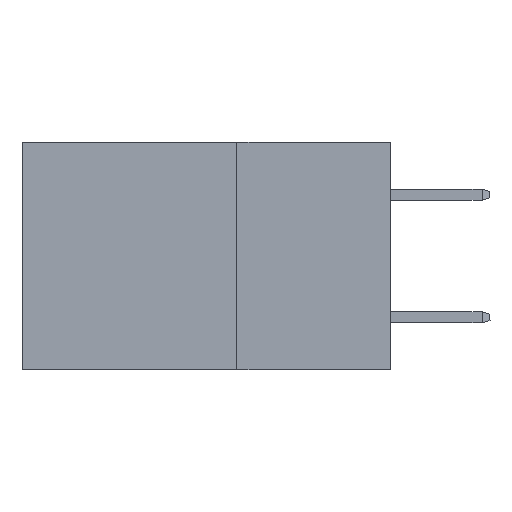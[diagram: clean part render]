
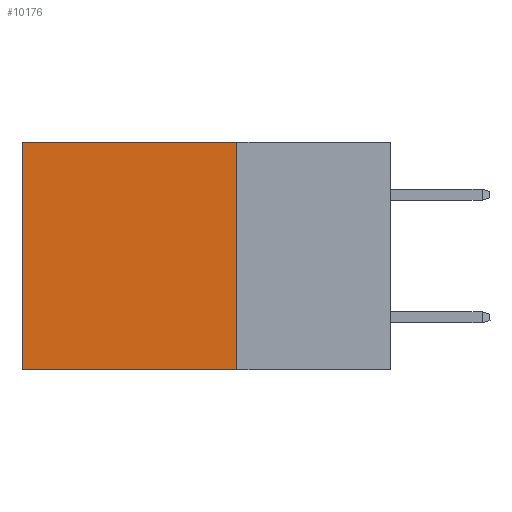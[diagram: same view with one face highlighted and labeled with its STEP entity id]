
A CAD part, left-side view. The second image highlights one B-rep face of the part: STEP entity #10176.
In plain terms, the highlighted planar face has unit normal (-1, 0, 0).
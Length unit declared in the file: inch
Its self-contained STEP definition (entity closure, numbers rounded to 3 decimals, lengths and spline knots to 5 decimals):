
#93 = VERTEX_POINT ( 'NONE', #11390 ) ;
#306 = VECTOR ( 'NONE', #2499, 39.37008 ) ;
#409 = EDGE_LOOP ( 'NONE', ( #2734, #11224, #6545, #11373 ) ) ;
#805 = LINE ( 'NONE', #5306, #1109 ) ;
#1109 = VECTOR ( 'NONE', #12263, 39.37008 ) ;
#1294 = VERTEX_POINT ( 'NONE', #9379 ) ;
#1542 = CARTESIAN_POINT ( 'NONE',  ( 0.2875, 0.6, 0. ) ) ;
#1719 = VECTOR ( 'NONE', #6880, 39.37008 ) ;
#2499 = DIRECTION ( 'NONE',  ( 0., 0., -1. ) ) ;
#2734 = ORIENTED_EDGE ( 'NONE', *, *, #5481, .T. ) ;
#2967 = AXIS2_PLACEMENT_3D ( 'NONE', #5669, #12609, #6627 ) ;
#3653 = LINE ( 'NONE', #11385, #8537 ) ;
#4625 = LINE ( 'NONE', #5899, #1719 ) ;
#4722 = VERTEX_POINT ( 'NONE', #7686 ) ;
#5306 = CARTESIAN_POINT ( 'NONE',  ( 0.2875, 0.25, -0.37 ) ) ;
#5342 = VERTEX_POINT ( 'NONE', #10679 ) ;
#5481 = EDGE_CURVE ( 'NONE', #1294, #4722, #8076, .T. ) ;
#5669 = CARTESIAN_POINT ( 'NONE',  ( 0.2875, 0.25, 0. ) ) ;
#5899 = CARTESIAN_POINT ( 'NONE',  ( 0.2875, 0.25, 0. ) ) ;
#6545 = ORIENTED_EDGE ( 'NONE', *, *, #6557, .F. ) ;
#6557 = EDGE_CURVE ( 'NONE', #5342, #93, #3653, .T. ) ;
#6627 = DIRECTION ( 'NONE',  ( 0., 0., -1. ) ) ;
#6880 = DIRECTION ( 'NONE',  ( 0., 1., 0. ) ) ;
#7686 = CARTESIAN_POINT ( 'NONE',  ( 0.2875, 0.6, -0.37 ) ) ;
#8076 = LINE ( 'NONE', #1542, #306 ) ;
#8537 = VECTOR ( 'NONE', #12393, 39.37008 ) ;
#9379 = CARTESIAN_POINT ( 'NONE',  ( 0.2875, 0.6, 0. ) ) ;
#10176 = ADVANCED_FACE ( 'NONE', ( #11137 ), #11626, .F. ) ;
#10679 = CARTESIAN_POINT ( 'NONE',  ( 0.2875, 0.25, 0. ) ) ;
#11137 = FACE_OUTER_BOUND ( 'NONE', #409, .T. ) ;
#11224 = ORIENTED_EDGE ( 'NONE', *, *, #12107, .F. ) ;
#11373 = ORIENTED_EDGE ( 'NONE', *, *, #12541, .T. ) ;
#11385 = CARTESIAN_POINT ( 'NONE',  ( 0.2875, 0.25, 0. ) ) ;
#11390 = CARTESIAN_POINT ( 'NONE',  ( 0.2875, 0.25, -0.37 ) ) ;
#11626 = PLANE ( 'NONE',  #2967 ) ;
#12107 = EDGE_CURVE ( 'NONE', #93, #4722, #805, .T. ) ;
#12263 = DIRECTION ( 'NONE',  ( 0., 1., 0. ) ) ;
#12393 = DIRECTION ( 'NONE',  ( 0., 0., -1. ) ) ;
#12541 = EDGE_CURVE ( 'NONE', #5342, #1294, #4625, .T. ) ;
#12609 = DIRECTION ( 'NONE',  ( 1., 0., 0. ) ) ;
